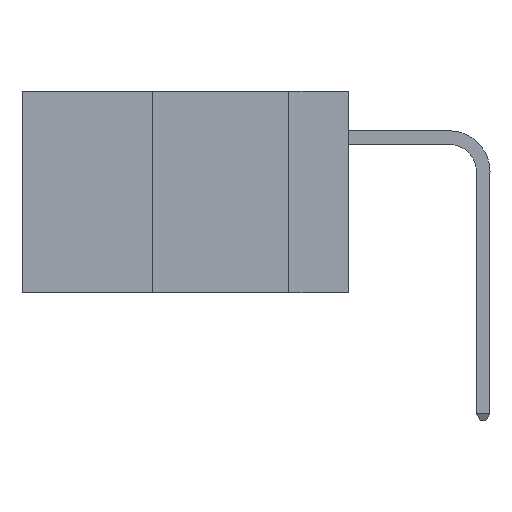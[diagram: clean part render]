
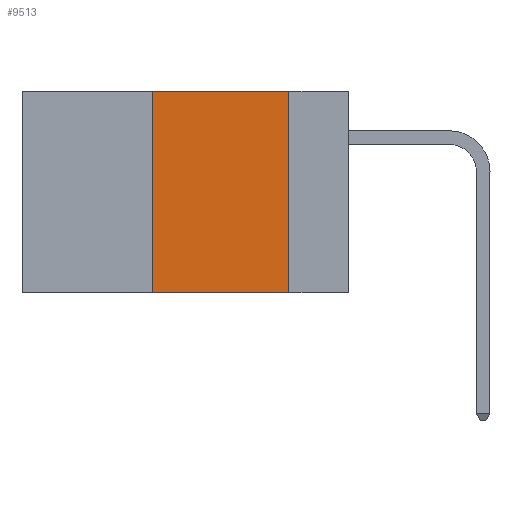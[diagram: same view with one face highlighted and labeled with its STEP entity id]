
A CAD part, left-side view. The second image highlights one B-rep face of the part: STEP entity #9513.
In plain terms, the highlighted planar face has unit normal (-1, 0, 0).
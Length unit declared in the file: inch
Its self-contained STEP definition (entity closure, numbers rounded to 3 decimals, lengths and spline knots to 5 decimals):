
#464 = VECTOR ( 'NONE', #13047, 39.37008 ) ;
#1445 = EDGE_CURVE ( 'NONE', #8530, #12736, #10313, .T. ) ;
#2114 = DIRECTION ( 'NONE',  ( 0., -1., 0. ) ) ;
#2401 = VECTOR ( 'NONE', #7000, 39.37008 ) ;
#2735 = LINE ( 'NONE', #8970, #2401 ) ;
#3069 = EDGE_CURVE ( 'NONE', #4339, #8530, #2735, .T. ) ;
#3107 = CARTESIAN_POINT ( 'NONE',  ( 0., 0.36, -0.37 ) ) ;
#3495 = AXIS2_PLACEMENT_3D ( 'NONE', #6825, #8954, #3608 ) ;
#3608 = DIRECTION ( 'NONE',  ( 0., 0., -1. ) ) ;
#4100 = ORIENTED_EDGE ( 'NONE', *, *, #12223, .F. ) ;
#4339 = VERTEX_POINT ( 'NONE', #3107 ) ;
#4652 = VECTOR ( 'NONE', #2114, 39.37008 ) ;
#5259 = ORIENTED_EDGE ( 'NONE', *, *, #3069, .F. ) ;
#5582 = CARTESIAN_POINT ( 'NONE',  ( 0., 0.6, -0.37 ) ) ;
#6806 = CARTESIAN_POINT ( 'NONE',  ( 0., 0.36, 0. ) ) ;
#6825 = CARTESIAN_POINT ( 'NONE',  ( 0., 0.6, 0. ) ) ;
#7000 = DIRECTION ( 'NONE',  ( 0., 0., 1. ) ) ;
#7617 = CARTESIAN_POINT ( 'NONE',  ( 0., 0.11, 0. ) ) ;
#7872 = EDGE_LOOP ( 'NONE', ( #4100, #10665, #5259, #13105 ) ) ;
#8530 = VERTEX_POINT ( 'NONE', #6806 ) ;
#8841 = LINE ( 'NONE', #7617, #12686 ) ;
#8954 = DIRECTION ( 'NONE',  ( 1., 0., 0. ) ) ;
#8970 = CARTESIAN_POINT ( 'NONE',  ( 0., 0.36, 0. ) ) ;
#9007 = VERTEX_POINT ( 'NONE', #13363 ) ;
#9048 = FACE_OUTER_BOUND ( 'NONE', #7872, .T. ) ;
#9513 = ADVANCED_FACE ( 'NONE', ( #9048 ), #12122, .F. ) ;
#10313 = LINE ( 'NONE', #11867, #4652 ) ;
#10627 = EDGE_CURVE ( 'NONE', #4339, #9007, #10686, .T. ) ;
#10665 = ORIENTED_EDGE ( 'NONE', *, *, #1445, .F. ) ;
#10686 = LINE ( 'NONE', #5582, #464 ) ;
#10761 = CARTESIAN_POINT ( 'NONE',  ( 0., 0.11, 0. ) ) ;
#11867 = CARTESIAN_POINT ( 'NONE',  ( 0., 0.6, 0. ) ) ;
#11888 = DIRECTION ( 'NONE',  ( 0., 0., -1. ) ) ;
#12122 = PLANE ( 'NONE',  #3495 ) ;
#12223 = EDGE_CURVE ( 'NONE', #12736, #9007, #8841, .T. ) ;
#12686 = VECTOR ( 'NONE', #11888, 39.37008 ) ;
#12736 = VERTEX_POINT ( 'NONE', #10761 ) ;
#13047 = DIRECTION ( 'NONE',  ( 0., -1., 0. ) ) ;
#13105 = ORIENTED_EDGE ( 'NONE', *, *, #10627, .T. ) ;
#13363 = CARTESIAN_POINT ( 'NONE',  ( 0., 0.11, -0.37 ) ) ;
